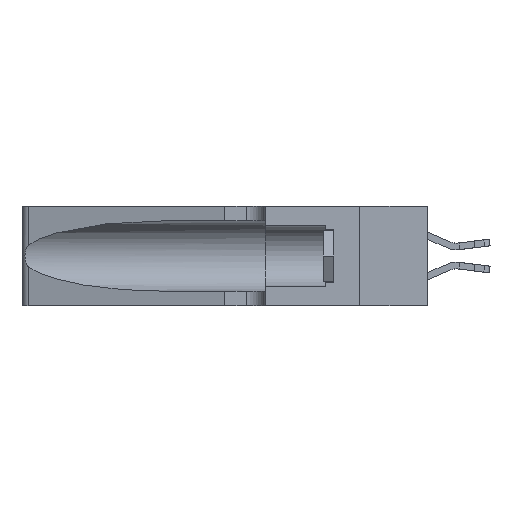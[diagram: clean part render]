
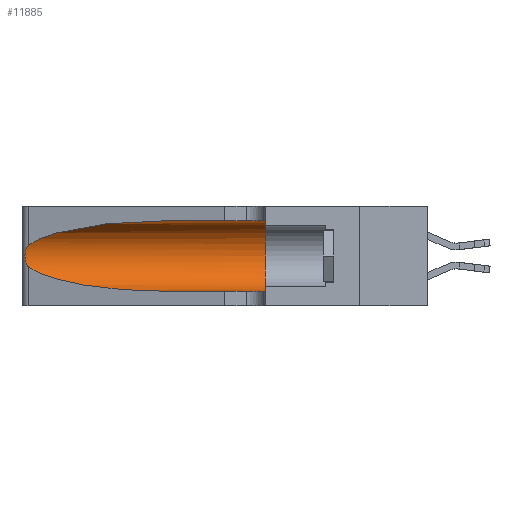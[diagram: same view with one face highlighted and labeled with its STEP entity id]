
A CAD part, left-side view. The second image highlights one B-rep face of the part: STEP entity #11885.
In plain terms, the highlighted cylindrical face has radius 3.308 mm (diameter 6.617 mm), a partial arc.
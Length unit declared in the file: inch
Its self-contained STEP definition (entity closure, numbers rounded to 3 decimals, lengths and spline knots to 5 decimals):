
#801 = CARTESIAN_POINT ( 'NONE',  ( 0.1305, 0.35, 0.05475 ) ) ;
#1317 = VERTEX_POINT ( 'NONE', #22221 ) ;
#1463 = ORIENTED_EDGE ( 'NONE', *, *, #22541, .F. ) ;
#2716 = CIRCLE ( 'NONE', #17091, 0.13025 ) ;
#2723 = CARTESIAN_POINT ( 'NONE',  ( 0.26017, 1.23833, 0.17102 ) ) ;
#2815 = DIRECTION ( 'NONE',  ( 0., 0., -1. ) ) ;
#2858 = VERTEX_POINT ( 'NONE', #801 ) ;
#2881 = CARTESIAN_POINT ( 'NONE',  ( 0.25639, 1.23186, 0.15144 ) ) ;
#2911 = DIRECTION ( 'NONE',  ( 0., 1., 0. ) ) ;
#3022 = DIRECTION ( 'NONE',  ( 0., -1., 0. ) ) ;
#3913 = LINE ( 'NONE', #11406, #12815 ) ;
#4069 = VERTEX_POINT ( 'NONE', #10336 ) ;
#4111 = CARTESIAN_POINT ( 'NONE',  ( 0.1305, 0.35, 0.31525 ) ) ;
#5550 = VERTEX_POINT ( 'NONE', #15033 ) ;
#6127 = DIRECTION ( 'NONE',  ( 0., -1., 0. ) ) ;
#6229 = VECTOR ( 'NONE', #3022, 39.37008 ) ;
#6613 = CARTESIAN_POINT ( 'NONE',  ( 0.18966, 0.96281, 0.05475 ) ) ;
#7297 = EDGE_LOOP ( 'NONE', ( #10448, #19858, #8609, #8641, #1463, #18083 ) ) ;
#7661 = EDGE_CURVE ( 'NONE', #1317, #4069, #13618, .T. ) ;
#7970 = EDGE_CURVE ( 'NONE', #4069, #2858, #3913, .T. ) ;
#8005 = CARTESIAN_POINT ( 'NONE',  ( 0.26018, 1.23835, 0.19895 ) ) ;
#8091 = CARTESIAN_POINT ( 'NONE',  ( 0.25487, 1.22718, 0.14631 ) ) ;
#8096 = CYLINDRICAL_SURFACE ( 'NONE', #19227, 0.13025 ) ;
#8609 = ORIENTED_EDGE ( 'NONE', *, *, #7661, .T. ) ;
#8641 = ORIENTED_EDGE ( 'NONE', *, *, #7970, .T. ) ;
#9868 = CARTESIAN_POINT ( 'NONE',  ( 0.26075, 1.23896, 0.19203 ) ) ;
#9882 = CARTESIAN_POINT ( 'NONE',  ( 0.2373, 1.15595, 0.08982 ) ) ;
#9945 = CARTESIAN_POINT ( 'NONE',  ( 0.25854, 1.2359, 0.20912 ) ) ;
#10188 = CARTESIAN_POINT ( 'NONE',  ( 0.25487, 1.22718, 0.14631 ) ) ;
#10336 = CARTESIAN_POINT ( 'NONE',  ( 0.1305, 0.72297, 0.05475 ) ) ;
#10448 = ORIENTED_EDGE ( 'NONE', *, *, #11728, .T. ) ;
#11193 = B_SPLINE_CURVE_WITH_KNOTS ( 'NONE', 3,
 ( #16983, #11811, #13441, #20692, #9945, #8005, #9868, #20616, #2723, #17203, #15348, #2881, #18737, #8091 ),
 .UNSPECIFIED., .F., .F.,
 ( 4, 2, 2, 2, 2, 2, 4 ),
 ( 0., 0.00027, 0.00053, 0.00107, 0.0016, 0.00187, 0.00214 ),
 .UNSPECIFIED. ) ;
#11406 = CARTESIAN_POINT ( 'NONE',  ( 0.1305, 1.61858, 0.05475 ) ) ;
#11728 = EDGE_CURVE ( 'NONE', #5550, #16594, #12190, .T. ) ;
#11811 = CARTESIAN_POINT ( 'NONE',  ( 0.25555, 1.22994, 0.2215 ) ) ;
#11885 = ADVANCED_FACE ( 'NONE', ( #19766 ), #8096, .F. ) ;
#12190 =( BOUNDED_CURVE ( )  B_SPLINE_CURVE ( 3, ( #17871, #21371, #20524, #22332 ),
 .UNSPECIFIED., .F., .T. ) 
 B_SPLINE_CURVE_WITH_KNOTS ( ( 4, 4 ),
 ( 1.5708, 2.84003 ),
 .UNSPECIFIED. ) 
 CURVE ( )  GEOMETRIC_REPRESENTATION_ITEM ( )  RATIONAL_B_SPLINE_CURVE ( ( 1., 0.87, 0.87, 1. ) ) 
 REPRESENTATION_ITEM ( '' )  );
#12815 = VECTOR ( 'NONE', #15004, 39.37008 ) ;
#13441 = CARTESIAN_POINT ( 'NONE',  ( 0.25639, 1.23184, 0.21858 ) ) ;
#13618 =( BOUNDED_CURVE ( )  B_SPLINE_CURVE ( 3, ( #10188, #9882, #6613, #17070 ),
 .UNSPECIFIED., .F., .F. ) 
 B_SPLINE_CURVE_WITH_KNOTS ( ( 4, 4 ),
 ( 3.44316, 4.71239 ),
 .UNSPECIFIED. ) 
 CURVE ( )  GEOMETRIC_REPRESENTATION_ITEM ( )  RATIONAL_B_SPLINE_CURVE ( ( 1., 0.87, 0.87, 1. ) ) 
 REPRESENTATION_ITEM ( '' )  );
#13780 = DIRECTION ( 'NONE',  ( 0., 0., 1. ) ) ;
#15004 = DIRECTION ( 'NONE',  ( 0., -1., 0. ) ) ;
#15033 = CARTESIAN_POINT ( 'NONE',  ( 0.1305, 0.72297, 0.31525 ) ) ;
#15348 = CARTESIAN_POINT ( 'NONE',  ( 0.25789, 1.23486, 0.15765 ) ) ;
#15625 = EDGE_CURVE ( 'NONE', #16594, #1317, #11193, .T. ) ;
#15996 = CARTESIAN_POINT ( 'NONE',  ( 0.25487, 1.22718, 0.22369 ) ) ;
#16594 = VERTEX_POINT ( 'NONE', #15996 ) ;
#16983 = CARTESIAN_POINT ( 'NONE',  ( 0.25487, 1.22718, 0.22369 ) ) ;
#17070 = CARTESIAN_POINT ( 'NONE',  ( 0.1305, 0.72297, 0.05475 ) ) ;
#17091 = AXIS2_PLACEMENT_3D ( 'NONE', #20951, #2911, #13780 ) ;
#17203 = CARTESIAN_POINT ( 'NONE',  ( 0.25856, 1.23593, 0.16098 ) ) ;
#17262 = VERTEX_POINT ( 'NONE', #4111 ) ;
#17871 = CARTESIAN_POINT ( 'NONE',  ( 0.1305, 0.72297, 0.31525 ) ) ;
#18083 = ORIENTED_EDGE ( 'NONE', *, *, #18708, .F. ) ;
#18708 = EDGE_CURVE ( 'NONE', #5550, #17262, #21551, .T. ) ;
#18737 = CARTESIAN_POINT ( 'NONE',  ( 0.25555, 1.22993, 0.14849 ) ) ;
#18747 = CARTESIAN_POINT ( 'NONE',  ( 0.1305, 1.61858, 0.185 ) ) ;
#18970 = CARTESIAN_POINT ( 'NONE',  ( 0.1305, 1.61858, 0.31525 ) ) ;
#19227 = AXIS2_PLACEMENT_3D ( 'NONE', #18747, #6127, #2815 ) ;
#19766 = FACE_OUTER_BOUND ( 'NONE', #7297, .T. ) ;
#19858 = ORIENTED_EDGE ( 'NONE', *, *, #15625, .T. ) ;
#20524 = CARTESIAN_POINT ( 'NONE',  ( 0.2373, 1.15595, 0.28018 ) ) ;
#20616 = CARTESIAN_POINT ( 'NONE',  ( 0.26075, 1.23896, 0.178 ) ) ;
#20692 = CARTESIAN_POINT ( 'NONE',  ( 0.25787, 1.23484, 0.2124 ) ) ;
#20951 = CARTESIAN_POINT ( 'NONE',  ( 0.1305, 0.35, 0.185 ) ) ;
#21371 = CARTESIAN_POINT ( 'NONE',  ( 0.18966, 0.96281, 0.31525 ) ) ;
#21551 = LINE ( 'NONE', #18970, #6229 ) ;
#22221 = CARTESIAN_POINT ( 'NONE',  ( 0.25487, 1.22718, 0.14631 ) ) ;
#22332 = CARTESIAN_POINT ( 'NONE',  ( 0.25487, 1.22718, 0.22369 ) ) ;
#22541 = EDGE_CURVE ( 'NONE', #17262, #2858, #2716, .T. ) ;
